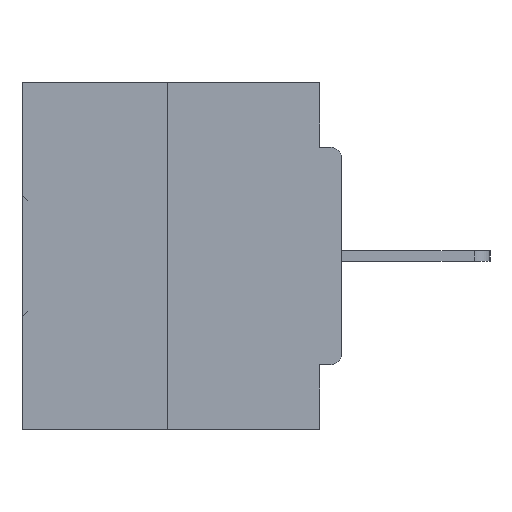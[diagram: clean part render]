
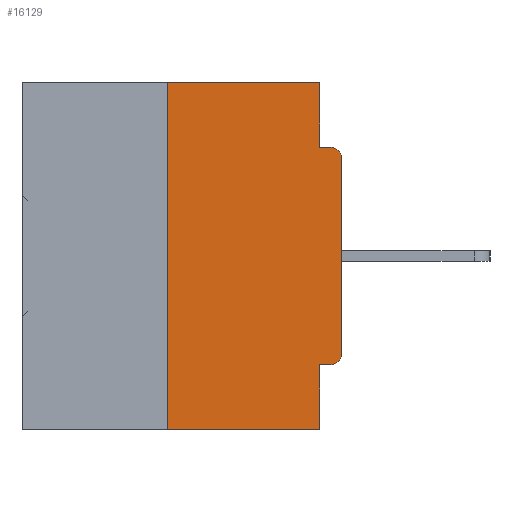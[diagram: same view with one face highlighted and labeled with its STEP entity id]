
A CAD part, left-side view. The second image highlights one B-rep face of the part: STEP entity #16129.
In plain terms, the highlighted planar face has unit normal (-1, 0, 0).
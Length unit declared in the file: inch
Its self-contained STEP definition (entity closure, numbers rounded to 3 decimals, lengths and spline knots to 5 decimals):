
#82 = VERTEX_POINT ( 'NONE', #15459 ) ;
#507 = CARTESIAN_POINT ( 'NONE',  ( 0., 0.25, 0. ) ) ;
#736 = CARTESIAN_POINT ( 'NONE',  ( 0., 0.015, -0.3915 ) ) ;
#1331 = DIRECTION ( 'NONE',  ( 0., -1., 0. ) ) ;
#1571 = CARTESIAN_POINT ( 'NONE',  ( 0., 0.031, -0.0935 ) ) ;
#1647 = VECTOR ( 'NONE', #34887, 39.37008 ) ;
#1657 = VERTEX_POINT ( 'NONE', #25796 ) ;
#1699 = ORIENTED_EDGE ( 'NONE', *, *, #11124, .F. ) ;
#2052 = DIRECTION ( 'NONE',  ( 0., 0., -1. ) ) ;
#2062 = ORIENTED_EDGE ( 'NONE', *, *, #26496, .F. ) ;
#2462 = DIRECTION ( 'NONE',  ( 0., 1., 0. ) ) ;
#2592 = ORIENTED_EDGE ( 'NONE', *, *, #16215, .T. ) ;
#3715 = LINE ( 'NONE', #9417, #36484 ) ;
#3928 = LINE ( 'NONE', #37823, #37184 ) ;
#4616 = DIRECTION ( 'NONE',  ( 0., -1., 0. ) ) ;
#4661 = ORIENTED_EDGE ( 'NONE', *, *, #12965, .F. ) ;
#5024 = EDGE_CURVE ( 'NONE', #15762, #33373, #3928, .T. ) ;
#6042 = VERTEX_POINT ( 'NONE', #22756 ) ;
#6080 = VERTEX_POINT ( 'NONE', #33150 ) ;
#6282 = VERTEX_POINT ( 'NONE', #507 ) ;
#6638 = DIRECTION ( 'NONE',  ( 0., 0., -1. ) ) ;
#8069 = ORIENTED_EDGE ( 'NONE', *, *, #5024, .T. ) ;
#8205 = LINE ( 'NONE', #11096, #37505 ) ;
#8356 = CARTESIAN_POINT ( 'NONE',  ( 0., 0.015, -0.1085 ) ) ;
#8550 = EDGE_CURVE ( 'NONE', #6042, #39380, #18545, .T. ) ;
#8630 = CARTESIAN_POINT ( 'NONE',  ( 0., 0.46, 0. ) ) ;
#9171 = EDGE_CURVE ( 'NONE', #1657, #33874, #18616, .T. ) ;
#9417 = CARTESIAN_POINT ( 'NONE',  ( 0., 0.46, -0.5 ) ) ;
#9876 = CARTESIAN_POINT ( 'NONE',  ( 0., 0., -0.3915 ) ) ;
#11062 = AXIS2_PLACEMENT_3D ( 'NONE', #8630, #30803, #27332 ) ;
#11096 = CARTESIAN_POINT ( 'NONE',  ( 0., 0.25, 0. ) ) ;
#11124 = EDGE_CURVE ( 'NONE', #39380, #6080, #36152, .T. ) ;
#11243 = ORIENTED_EDGE ( 'NONE', *, *, #37788, .T. ) ;
#11551 = DIRECTION ( 'NONE',  ( -1., 0., 0. ) ) ;
#12767 = DIRECTION ( 'NONE',  ( 0., 0., 1. ) ) ;
#12907 = DIRECTION ( 'NONE',  ( -1., 0., 0. ) ) ;
#12965 = EDGE_CURVE ( 'NONE', #82, #6282, #8205, .T. ) ;
#13100 = DIRECTION ( 'NONE',  ( 0., 0., -1. ) ) ;
#14287 = EDGE_CURVE ( 'NONE', #17939, #1657, #35419, .T. ) ;
#15393 = DIRECTION ( 'NONE',  ( 0., -1., 0. ) ) ;
#15459 = CARTESIAN_POINT ( 'NONE',  ( 0., 0.25, -0.5 ) ) ;
#15561 = VECTOR ( 'NONE', #13100, 39.37008 ) ;
#15762 = VERTEX_POINT ( 'NONE', #9876 ) ;
#16129 = ADVANCED_FACE ( 'NONE', ( #22083 ), #33842, .F. ) ;
#16215 = EDGE_CURVE ( 'NONE', #82, #33874, #3715, .T. ) ;
#16743 = EDGE_CURVE ( 'NONE', #17939, #15762, #19068, .T. ) ;
#17084 = AXIS2_PLACEMENT_3D ( 'NONE', #8356, #11551, #2052 ) ;
#17939 = VERTEX_POINT ( 'NONE', #24709 ) ;
#18201 = CARTESIAN_POINT ( 'NONE',  ( 0., 0., -0.4065 ) ) ;
#18545 = LINE ( 'NONE', #32078, #15561 ) ;
#18616 = LINE ( 'NONE', #25185, #1647 ) ;
#19068 = CIRCLE ( 'NONE', #28716, 0.015 ) ;
#22083 = FACE_OUTER_BOUND ( 'NONE', #25792, .T. ) ;
#22756 = CARTESIAN_POINT ( 'NONE',  ( 0., 0.031, 0. ) ) ;
#23101 = LINE ( 'NONE', #23798, #35524 ) ;
#23301 = CARTESIAN_POINT ( 'NONE',  ( 0., 0., -0.0935 ) ) ;
#23514 = ORIENTED_EDGE ( 'NONE', *, *, #9171, .F. ) ;
#23518 = CARTESIAN_POINT ( 'NONE',  ( 0., 0.031, -0.5 ) ) ;
#23798 = CARTESIAN_POINT ( 'NONE',  ( 0., 0.46, 0. ) ) ;
#24709 = CARTESIAN_POINT ( 'NONE',  ( 0., 0.015, -0.4065 ) ) ;
#25185 = CARTESIAN_POINT ( 'NONE',  ( 0., 0.031, -0.5 ) ) ;
#25792 = EDGE_LOOP ( 'NONE', ( #2062, #4661, #2592, #23514, #35686, #30466, #8069, #11243, #1699, #26530 ) ) ;
#25796 = CARTESIAN_POINT ( 'NONE',  ( 0., 0.031, -0.4065 ) ) ;
#26480 = DIRECTION ( 'NONE',  ( 0., 0., 1. ) ) ;
#26496 = EDGE_CURVE ( 'NONE', #6282, #6042, #23101, .T. ) ;
#26530 = ORIENTED_EDGE ( 'NONE', *, *, #8550, .F. ) ;
#26771 = CARTESIAN_POINT ( 'NONE',  ( 0., 0., -0.1085 ) ) ;
#27332 = DIRECTION ( 'NONE',  ( 0., 0., -1. ) ) ;
#28716 = AXIS2_PLACEMENT_3D ( 'NONE', #736, #12907, #6638 ) ;
#30466 = ORIENTED_EDGE ( 'NONE', *, *, #16743, .T. ) ;
#30803 = DIRECTION ( 'NONE',  ( 1., 0., 0. ) ) ;
#32078 = CARTESIAN_POINT ( 'NONE',  ( 0., 0.031, 0. ) ) ;
#33150 = CARTESIAN_POINT ( 'NONE',  ( 0., 0.015, -0.0935 ) ) ;
#33373 = VERTEX_POINT ( 'NONE', #26771 ) ;
#33842 = PLANE ( 'NONE',  #11062 ) ;
#33874 = VERTEX_POINT ( 'NONE', #23518 ) ;
#34887 = DIRECTION ( 'NONE',  ( 0., 0., -1. ) ) ;
#34930 = VECTOR ( 'NONE', #2462, 39.37008 ) ;
#35419 = LINE ( 'NONE', #18201, #34930 ) ;
#35524 = VECTOR ( 'NONE', #4616, 39.37008 ) ;
#35686 = ORIENTED_EDGE ( 'NONE', *, *, #14287, .F. ) ;
#36152 = LINE ( 'NONE', #23301, #37614 ) ;
#36484 = VECTOR ( 'NONE', #15393, 39.37008 ) ;
#37184 = VECTOR ( 'NONE', #12767, 39.37008 ) ;
#37505 = VECTOR ( 'NONE', #26480, 39.37008 ) ;
#37614 = VECTOR ( 'NONE', #1331, 39.37008 ) ;
#37788 = EDGE_CURVE ( 'NONE', #33373, #6080, #40710, .T. ) ;
#37823 = CARTESIAN_POINT ( 'NONE',  ( 0., 0., 0. ) ) ;
#39380 = VERTEX_POINT ( 'NONE', #1571 ) ;
#40710 = CIRCLE ( 'NONE', #17084, 0.015 ) ;
